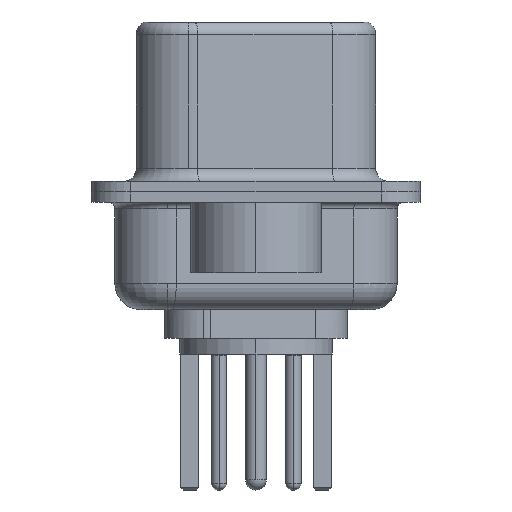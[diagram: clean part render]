
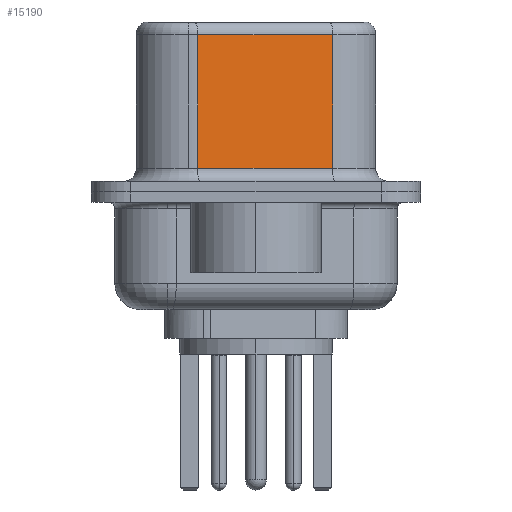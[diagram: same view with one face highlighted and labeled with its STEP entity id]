
A CAD part, left-side view. The second image highlights one B-rep face of the part: STEP entity #15190.
In plain terms, the highlighted planar face has unit normal (-0.985, -0.174, 0).
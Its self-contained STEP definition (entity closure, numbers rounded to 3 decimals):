
#690 = VERTEX_POINT ( 'NONE', #19149 ) ;
#751 = VECTOR ( 'NONE', #16789, 1000. ) ;
#1409 = CARTESIAN_POINT ( 'NONE',  ( 3.675, 2.233, 6.02 ) ) ;
#3045 = DIRECTION ( 'NONE',  ( 0., 0., -1. ) ) ;
#3048 = PLANE ( 'NONE',  #18316 ) ;
#3352 = CARTESIAN_POINT ( 'NONE',  ( 4.585, -2.927, 6.02 ) ) ;
#3449 = VECTOR ( 'NONE', #14380, 1000. ) ;
#3500 = EDGE_CURVE ( 'NONE', #690, #9549, #14621, .T. ) ;
#3955 = EDGE_CURVE ( 'NONE', #12908, #6304, #8061, .T. ) ;
#4606 = ORIENTED_EDGE ( 'NONE', *, *, #4637, .F. ) ;
#4637 = EDGE_CURVE ( 'NONE', #12908, #9549, #19665, .T. ) ;
#5438 = CARTESIAN_POINT ( 'NONE',  ( 4.585, -2.927, 0.9 ) ) ;
#6304 = VERTEX_POINT ( 'NONE', #1409 ) ;
#6503 = DIRECTION ( 'NONE',  ( -0.174, 0.985, 0. ) ) ;
#6608 = LINE ( 'NONE', #11825, #19888 ) ;
#7254 = EDGE_CURVE ( 'NONE', #6304, #690, #6608, .T. ) ;
#8061 = LINE ( 'NONE', #12354, #3449 ) ;
#8158 = ORIENTED_EDGE ( 'NONE', *, *, #3955, .T. ) ;
#9439 = FACE_OUTER_BOUND ( 'NONE', #13369, .T. ) ;
#9549 = VERTEX_POINT ( 'NONE', #5438 ) ;
#11825 = CARTESIAN_POINT ( 'NONE',  ( 3.675, 2.233, 6.52 ) ) ;
#12354 = CARTESIAN_POINT ( 'NONE',  ( 4.585, -2.927, 6.02 ) ) ;
#12908 = VERTEX_POINT ( 'NONE', #3352 ) ;
#13369 = EDGE_LOOP ( 'NONE', ( #4606, #8158, #19119, #18591 ) ) ;
#14163 = CARTESIAN_POINT ( 'NONE',  ( 4.585, -2.927, 6.52 ) ) ;
#14380 = DIRECTION ( 'NONE',  ( -0.174, 0.985, 0. ) ) ;
#14621 = LINE ( 'NONE', #20545, #751 ) ;
#15111 = VECTOR ( 'NONE', #20849, 1000. ) ;
#15189 = CARTESIAN_POINT ( 'NONE',  ( 4.585, -2.927, 6.52 ) ) ;
#15190 = ADVANCED_FACE ( 'NONE', ( #9439 ), #3048, .F. ) ;
#16789 = DIRECTION ( 'NONE',  ( 0.174, -0.985, 0. ) ) ;
#16906 = DIRECTION ( 'NONE',  ( 0.985, 0.174, 0. ) ) ;
#18316 = AXIS2_PLACEMENT_3D ( 'NONE', #15189, #16906, #6503 ) ;
#18591 = ORIENTED_EDGE ( 'NONE', *, *, #3500, .T. ) ;
#19119 = ORIENTED_EDGE ( 'NONE', *, *, #7254, .T. ) ;
#19149 = CARTESIAN_POINT ( 'NONE',  ( 3.675, 2.233, 0.9 ) ) ;
#19665 = LINE ( 'NONE', #14163, #15111 ) ;
#19888 = VECTOR ( 'NONE', #3045, 1000. ) ;
#20545 = CARTESIAN_POINT ( 'NONE',  ( 4.585, -2.927, 0.9 ) ) ;
#20849 = DIRECTION ( 'NONE',  ( 0., 0., -1. ) ) ;
